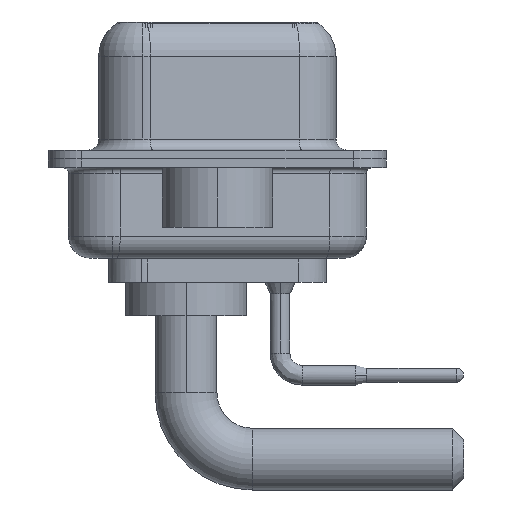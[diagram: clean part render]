
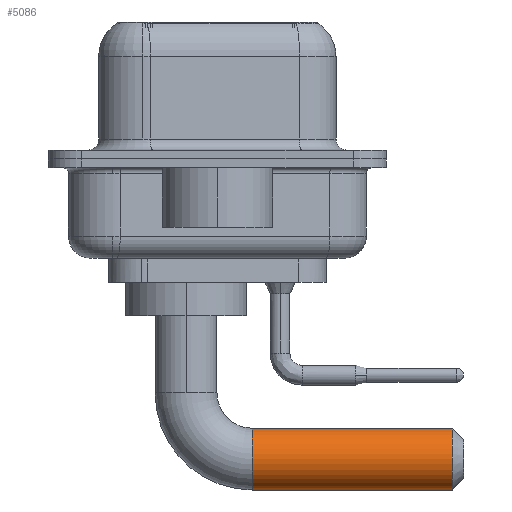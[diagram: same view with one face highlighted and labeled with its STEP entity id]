
A CAD part, left-side view. The second image highlights one B-rep face of the part: STEP entity #5086.
In plain terms, the highlighted cylindrical face has radius 1.4 mm (diameter 2.8 mm), a partial arc.
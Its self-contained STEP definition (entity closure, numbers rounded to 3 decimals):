
#1571 = EDGE_CURVE ( 'NONE', #10607, #5121, #16415, .T. ) ;
#1706 = AXIS2_PLACEMENT_3D ( 'NONE', #4154, #9443, #15889 ) ;
#3314 = EDGE_CURVE ( 'NONE', #5530, #4980, #16822, .T. ) ;
#4154 = CARTESIAN_POINT ( 'NONE',  ( 0., -12.07, -6.5 ) ) ;
#4431 = CARTESIAN_POINT ( 'NONE',  ( 0., -3., -7.9 ) ) ;
#4724 = DIRECTION ( 'NONE',  ( 0., -1., 0. ) ) ;
#4855 = DIRECTION ( 'NONE',  ( 0., -1., 0. ) ) ;
#4980 = VERTEX_POINT ( 'NONE', #9764 ) ;
#5086 = ADVANCED_FACE ( 'NONE', ( #6964 ), #12136, .T. ) ;
#5121 = VERTEX_POINT ( 'NONE', #7170 ) ;
#5270 = ORIENTED_EDGE ( 'NONE', *, *, #7457, .T. ) ;
#5530 = VERTEX_POINT ( 'NONE', #9267 ) ;
#5931 = ORIENTED_EDGE ( 'NONE', *, *, #9405, .F. ) ;
#6792 = DIRECTION ( 'NONE',  ( 0., -1., 0. ) ) ;
#6852 = DIRECTION ( 'NONE',  ( 0., -1., 0. ) ) ;
#6964 = FACE_OUTER_BOUND ( 'NONE', #16599, .T. ) ;
#7170 = CARTESIAN_POINT ( 'NONE',  ( 0., -3., -7.9 ) ) ;
#7457 = EDGE_CURVE ( 'NONE', #5121, #5530, #19597, .T. ) ;
#8194 = CARTESIAN_POINT ( 'NONE',  ( 0., -3., -6.5 ) ) ;
#9267 = CARTESIAN_POINT ( 'NONE',  ( 0., -12.07, -7.9 ) ) ;
#9349 = AXIS2_PLACEMENT_3D ( 'NONE', #15032, #6852, #10191 ) ;
#9405 = EDGE_CURVE ( 'NONE', #10607, #4980, #10135, .T. ) ;
#9443 = DIRECTION ( 'NONE',  ( 0., 1., 0. ) ) ;
#9764 = CARTESIAN_POINT ( 'NONE',  ( 0., -12.07, -5.1 ) ) ;
#10135 = LINE ( 'NONE', #13468, #19124 ) ;
#10191 = DIRECTION ( 'NONE',  ( 0., 0., -1. ) ) ;
#10607 = VERTEX_POINT ( 'NONE', #20926 ) ;
#11317 = DIRECTION ( 'NONE',  ( -1., 0., 0. ) ) ;
#12136 = CYLINDRICAL_SURFACE ( 'NONE', #9349, 1.4 ) ;
#13468 = CARTESIAN_POINT ( 'NONE',  ( 0., -3., -5.1 ) ) ;
#13859 = VECTOR ( 'NONE', #4855, 1000. ) ;
#14035 = AXIS2_PLACEMENT_3D ( 'NONE', #8194, #4724, #11317 ) ;
#14440 = ORIENTED_EDGE ( 'NONE', *, *, #3314, .T. ) ;
#15032 = CARTESIAN_POINT ( 'NONE',  ( 0., -3., -6.5 ) ) ;
#15889 = DIRECTION ( 'NONE',  ( 0., 0., -1. ) ) ;
#16415 = CIRCLE ( 'NONE', #14035, 1.4 ) ;
#16599 = EDGE_LOOP ( 'NONE', ( #5931, #18521, #5270, #14440 ) ) ;
#16822 = CIRCLE ( 'NONE', #1706, 1.4 ) ;
#18521 = ORIENTED_EDGE ( 'NONE', *, *, #1571, .T. ) ;
#19124 = VECTOR ( 'NONE', #6792, 1000. ) ;
#19597 = LINE ( 'NONE', #4431, #13859 ) ;
#20926 = CARTESIAN_POINT ( 'NONE',  ( 0., -3., -5.1 ) ) ;
